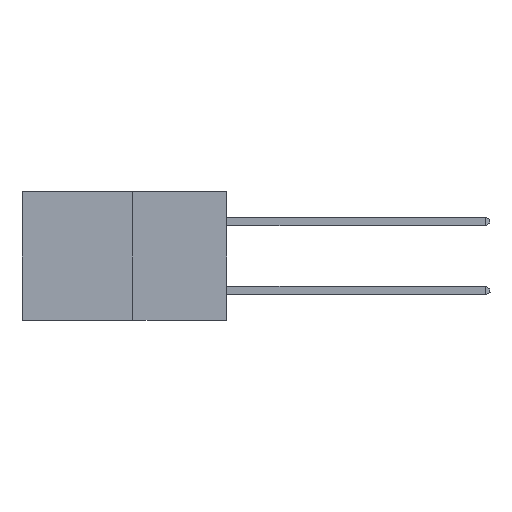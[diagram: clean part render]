
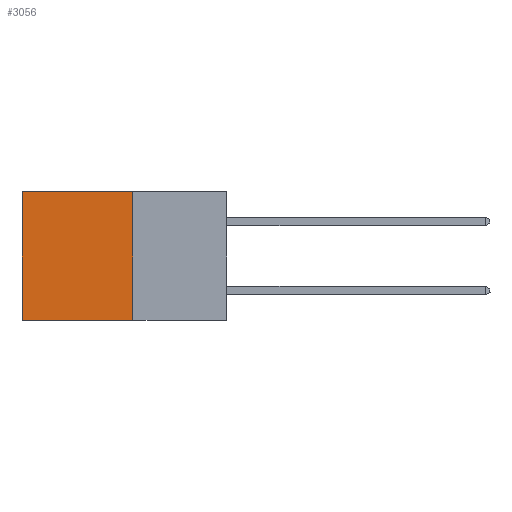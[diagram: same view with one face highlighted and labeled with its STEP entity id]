
A CAD part, left-side view. The second image highlights one B-rep face of the part: STEP entity #3056.
In plain terms, the highlighted planar face has unit normal (-1, 0, 0).
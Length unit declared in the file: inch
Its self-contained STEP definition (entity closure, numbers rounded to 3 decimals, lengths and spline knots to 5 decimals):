
#1361 = ORIENTED_EDGE ( 'NONE', *, *, #14671, .F. ) ;
#2114 = CARTESIAN_POINT ( 'NONE',  ( 0.277, 0.27, 0. ) ) ;
#2376 = PLANE ( 'NONE',  #11216 ) ;
#2411 = CARTESIAN_POINT ( 'NONE',  ( 0.277, 0.27, -0.37 ) ) ;
#2666 = VECTOR ( 'NONE', #3907, 39.37008 ) ;
#3056 = ADVANCED_FACE ( 'NONE', ( #18731 ), #2376, .F. ) ;
#3907 = DIRECTION ( 'NONE',  ( 0., 0., -1. ) ) ;
#4069 = EDGE_LOOP ( 'NONE', ( #10386, #1361, #11695, #5518 ) ) ;
#4428 = VERTEX_POINT ( 'NONE', #18169 ) ;
#4647 = LINE ( 'NONE', #13105, #20839 ) ;
#5518 = ORIENTED_EDGE ( 'NONE', *, *, #20262, .T. ) ;
#6611 = DIRECTION ( 'NONE',  ( 0., 1., 0. ) ) ;
#6719 = CARTESIAN_POINT ( 'NONE',  ( 0.277, 0.27, -0.37 ) ) ;
#7052 = LINE ( 'NONE', #12122, #2666 ) ;
#7196 = EDGE_CURVE ( 'NONE', #18575, #4428, #9394, .T. ) ;
#7385 = DIRECTION ( 'NONE',  ( 0., 1., 0. ) ) ;
#8209 = VECTOR ( 'NONE', #7385, 39.37008 ) ;
#9394 = LINE ( 'NONE', #6719, #17480 ) ;
#9689 = DIRECTION ( 'NONE',  ( 0., 0., -1. ) ) ;
#10386 = ORIENTED_EDGE ( 'NONE', *, *, #18650, .T. ) ;
#11216 = AXIS2_PLACEMENT_3D ( 'NONE', #12277, #19316, #19247 ) ;
#11695 = ORIENTED_EDGE ( 'NONE', *, *, #7196, .F. ) ;
#12122 = CARTESIAN_POINT ( 'NONE',  ( 0.277, 0.59, -0.37 ) ) ;
#12277 = CARTESIAN_POINT ( 'NONE',  ( 0.277, 0.27, -0.37 ) ) ;
#12513 = LINE ( 'NONE', #2411, #8209 ) ;
#13105 = CARTESIAN_POINT ( 'NONE',  ( 0.277, 0.27, 0. ) ) ;
#14671 = EDGE_CURVE ( 'NONE', #4428, #19778, #12513, .T. ) ;
#17085 = CARTESIAN_POINT ( 'NONE',  ( 0.277, 0.59, 0. ) ) ;
#17480 = VECTOR ( 'NONE', #9689, 39.37008 ) ;
#18169 = CARTESIAN_POINT ( 'NONE',  ( 0.277, 0.27, -0.37 ) ) ;
#18575 = VERTEX_POINT ( 'NONE', #2114 ) ;
#18650 = EDGE_CURVE ( 'NONE', #19194, #19778, #7052, .T. ) ;
#18731 = FACE_OUTER_BOUND ( 'NONE', #4069, .T. ) ;
#19194 = VERTEX_POINT ( 'NONE', #17085 ) ;
#19247 = DIRECTION ( 'NONE',  ( 0., 0., -1. ) ) ;
#19316 = DIRECTION ( 'NONE',  ( 1., 0., 0. ) ) ;
#19778 = VERTEX_POINT ( 'NONE', #20045 ) ;
#20045 = CARTESIAN_POINT ( 'NONE',  ( 0.277, 0.59, -0.37 ) ) ;
#20262 = EDGE_CURVE ( 'NONE', #18575, #19194, #4647, .T. ) ;
#20839 = VECTOR ( 'NONE', #6611, 39.37008 ) ;
